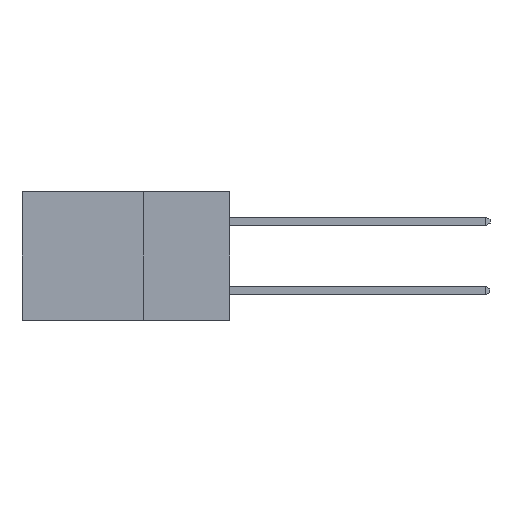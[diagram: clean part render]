
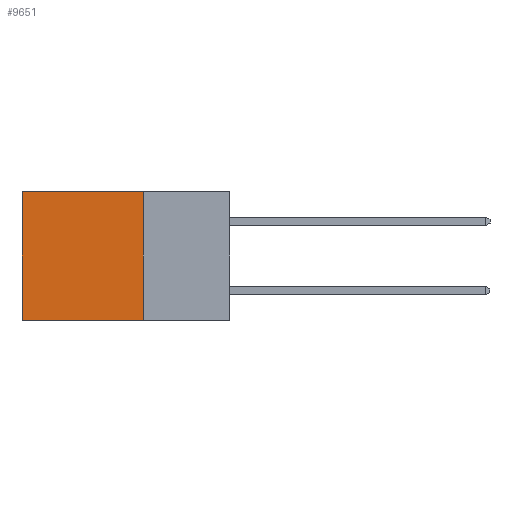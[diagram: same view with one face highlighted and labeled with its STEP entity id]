
A CAD part, left-side view. The second image highlights one B-rep face of the part: STEP entity #9651.
In plain terms, the highlighted planar face has unit normal (-1, 0, 0).
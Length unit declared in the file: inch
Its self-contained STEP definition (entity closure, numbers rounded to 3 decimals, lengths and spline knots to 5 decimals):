
#432 = VERTEX_POINT ( 'NONE', #1346 ) ;
#466 = VECTOR ( 'NONE', #8818, 39.37008 ) ;
#967 = CARTESIAN_POINT ( 'NONE',  ( 0.298, 0.25, -0.37 ) ) ;
#1346 = CARTESIAN_POINT ( 'NONE',  ( 0.298, 0.6, -0.37 ) ) ;
#1569 = VECTOR ( 'NONE', #6331, 39.37008 ) ;
#2768 = EDGE_CURVE ( 'NONE', #4375, #432, #7612, .T. ) ;
#3558 = CARTESIAN_POINT ( 'NONE',  ( 0.298, 0.6, 0. ) ) ;
#3646 = VECTOR ( 'NONE', #5707, 39.37008 ) ;
#3680 = VERTEX_POINT ( 'NONE', #13491 ) ;
#4252 = VERTEX_POINT ( 'NONE', #967 ) ;
#4375 = VERTEX_POINT ( 'NONE', #11161 ) ;
#4657 = ORIENTED_EDGE ( 'NONE', *, *, #9913, .T. ) ;
#5006 = LINE ( 'NONE', #12630, #10824 ) ;
#5615 = CARTESIAN_POINT ( 'NONE',  ( 0.298, 0.25, 0. ) ) ;
#5707 = DIRECTION ( 'NONE',  ( 0., 1., 0. ) ) ;
#6123 = AXIS2_PLACEMENT_3D ( 'NONE', #7447, #7430, #7415 ) ;
#6258 = ORIENTED_EDGE ( 'NONE', *, *, #14155, .F. ) ;
#6331 = DIRECTION ( 'NONE',  ( 0., 0., -1. ) ) ;
#7415 = DIRECTION ( 'NONE',  ( 0., 0., -1. ) ) ;
#7430 = DIRECTION ( 'NONE',  ( 1., 0., 0. ) ) ;
#7447 = CARTESIAN_POINT ( 'NONE',  ( 0.298, 0.25, 0. ) ) ;
#7612 = LINE ( 'NONE', #3558, #1569 ) ;
#7673 = PLANE ( 'NONE',  #6123 ) ;
#8221 = EDGE_CURVE ( 'NONE', #3680, #4252, #10686, .T. ) ;
#8818 = DIRECTION ( 'NONE',  ( 0., 0., -1. ) ) ;
#9163 = CARTESIAN_POINT ( 'NONE',  ( 0.298, 0.25, 0. ) ) ;
#9651 = ADVANCED_FACE ( 'NONE', ( #10444 ), #7673, .F. ) ;
#9899 = LINE ( 'NONE', #5615, #3646 ) ;
#9913 = EDGE_CURVE ( 'NONE', #3680, #4375, #9899, .T. ) ;
#10113 = EDGE_LOOP ( 'NONE', ( #13856, #6258, #14997, #4657 ) ) ;
#10444 = FACE_OUTER_BOUND ( 'NONE', #10113, .T. ) ;
#10686 = LINE ( 'NONE', #9163, #466 ) ;
#10824 = VECTOR ( 'NONE', #13769, 39.37008 ) ;
#11161 = CARTESIAN_POINT ( 'NONE',  ( 0.298, 0.6, 0. ) ) ;
#12630 = CARTESIAN_POINT ( 'NONE',  ( 0.298, 0.25, -0.37 ) ) ;
#13491 = CARTESIAN_POINT ( 'NONE',  ( 0.298, 0.25, 0. ) ) ;
#13769 = DIRECTION ( 'NONE',  ( 0., 1., 0. ) ) ;
#13856 = ORIENTED_EDGE ( 'NONE', *, *, #2768, .T. ) ;
#14155 = EDGE_CURVE ( 'NONE', #4252, #432, #5006, .T. ) ;
#14997 = ORIENTED_EDGE ( 'NONE', *, *, #8221, .F. ) ;
